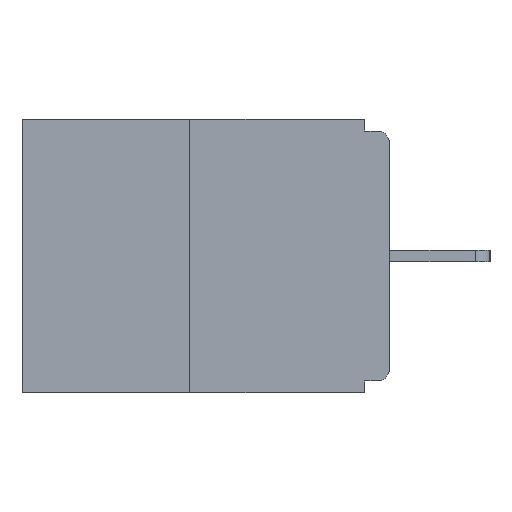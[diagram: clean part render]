
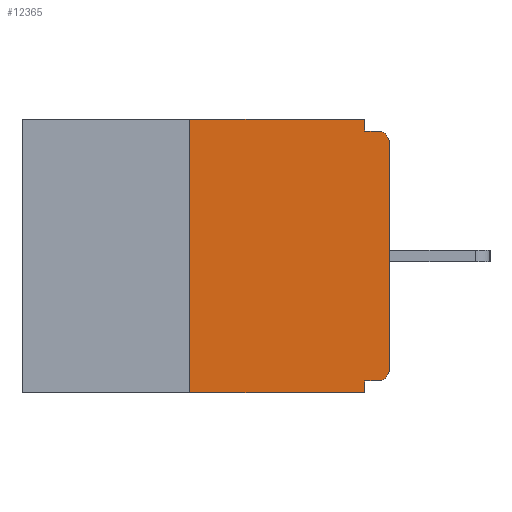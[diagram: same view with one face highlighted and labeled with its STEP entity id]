
A CAD part, left-side view. The second image highlights one B-rep face of the part: STEP entity #12365.
In plain terms, the highlighted planar face has unit normal (-1, 0, 0).
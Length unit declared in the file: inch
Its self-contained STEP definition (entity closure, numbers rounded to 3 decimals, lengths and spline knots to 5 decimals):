
#822 = DIRECTION ( 'NONE',  ( 0., 1., 0. ) ) ;
#905 = CARTESIAN_POINT ( 'NONE',  ( 0., 0.031, -0.015 ) ) ;
#998 = CARTESIAN_POINT ( 'NONE',  ( 0., 0.031, -0.343 ) ) ;
#1504 = DIRECTION ( 'NONE',  ( 0., -1., 0. ) ) ;
#1650 = VERTEX_POINT ( 'NONE', #905 ) ;
#1698 = CARTESIAN_POINT ( 'NONE',  ( 0., 0., -0.03 ) ) ;
#1766 = VERTEX_POINT ( 'NONE', #1698 ) ;
#1811 = EDGE_CURVE ( 'NONE', #2422, #1650, #21264, .T. ) ;
#2151 = EDGE_CURVE ( 'NONE', #22744, #8862, #3269, .T. ) ;
#2422 = VERTEX_POINT ( 'NONE', #18905 ) ;
#2938 = VECTOR ( 'NONE', #8432, 39.37008 ) ;
#3102 = EDGE_CURVE ( 'NONE', #8862, #6666, #23580, .T. ) ;
#3162 = CARTESIAN_POINT ( 'NONE',  ( 0., 0.015, -0.03 ) ) ;
#3269 = LINE ( 'NONE', #3898, #12607 ) ;
#3799 = LINE ( 'NONE', #23563, #12544 ) ;
#3820 = DIRECTION ( 'NONE',  ( 0., 0., -1. ) ) ;
#3898 = CARTESIAN_POINT ( 'NONE',  ( 0., 0., -0.328 ) ) ;
#4153 = DIRECTION ( 'NONE',  ( 0., 0., 1. ) ) ;
#4373 = EDGE_CURVE ( 'NONE', #10831, #6666, #16739, .T. ) ;
#4634 = EDGE_LOOP ( 'NONE', ( #5738, #5782, #6149, #6290, #6574, #6686, #6690, #6829, #7350, #7524 ) ) ;
#5040 = DIRECTION ( 'NONE',  ( 0., 0., -1. ) ) ;
#5623 = EDGE_CURVE ( 'NONE', #10831, #16930, #23477, .T. ) ;
#5738 = ORIENTED_EDGE ( 'NONE', *, *, #20176, .F. ) ;
#5782 = ORIENTED_EDGE ( 'NONE', *, *, #5623, .F. ) ;
#5790 = DIRECTION ( 'NONE',  ( 0., -1., 0. ) ) ;
#6149 = ORIENTED_EDGE ( 'NONE', *, *, #4373, .T. ) ;
#6290 = ORIENTED_EDGE ( 'NONE', *, *, #3102, .F. ) ;
#6547 = CARTESIAN_POINT ( 'NONE',  ( 0., 0., -0.015 ) ) ;
#6574 = ORIENTED_EDGE ( 'NONE', *, *, #2151, .F. ) ;
#6611 = VECTOR ( 'NONE', #22834, 39.37008 ) ;
#6666 = VERTEX_POINT ( 'NONE', #20913 ) ;
#6686 = ORIENTED_EDGE ( 'NONE', *, *, #17484, .T. ) ;
#6690 = ORIENTED_EDGE ( 'NONE', *, *, #7205, .T. ) ;
#6764 = DIRECTION ( 'NONE',  ( 0., 0., 1. ) ) ;
#6829 = ORIENTED_EDGE ( 'NONE', *, *, #15104, .T. ) ;
#7196 = CARTESIAN_POINT ( 'NONE',  ( 0., 0.46, 0. ) ) ;
#7205 = EDGE_CURVE ( 'NONE', #22937, #1766, #16019, .T. ) ;
#7350 = ORIENTED_EDGE ( 'NONE', *, *, #19973, .F. ) ;
#7524 = ORIENTED_EDGE ( 'NONE', *, *, #1811, .F. ) ;
#7939 = AXIS2_PLACEMENT_3D ( 'NONE', #3162, #16099, #5040 ) ;
#8432 = DIRECTION ( 'NONE',  ( 0., -1., 0. ) ) ;
#8862 = VERTEX_POINT ( 'NONE', #17153 ) ;
#8929 = FACE_OUTER_BOUND ( 'NONE', #4634, .T. ) ;
#8953 = DIRECTION ( 'NONE',  ( -1., 0., 0. ) ) ;
#9081 = DIRECTION ( 'NONE',  ( 0., 0., -1. ) ) ;
#10043 = CARTESIAN_POINT ( 'NONE',  ( 0., 0.25, -0.343 ) ) ;
#10435 = CARTESIAN_POINT ( 'NONE',  ( 0., 0.25, 0. ) ) ;
#10768 = VECTOR ( 'NONE', #5790, 39.37008 ) ;
#10831 = VERTEX_POINT ( 'NONE', #10043 ) ;
#12298 = CARTESIAN_POINT ( 'NONE',  ( 0., 0.25, 0. ) ) ;
#12365 = ADVANCED_FACE ( 'NONE', ( #8929 ), #12728, .F. ) ;
#12544 = VECTOR ( 'NONE', #1504, 39.37008 ) ;
#12607 = VECTOR ( 'NONE', #822, 39.37008 ) ;
#12728 = PLANE ( 'NONE',  #23051 ) ;
#12901 = CARTESIAN_POINT ( 'NONE',  ( 0., 0.031, 0. ) ) ;
#12955 = AXIS2_PLACEMENT_3D ( 'NONE', #19921, #8953, #21729 ) ;
#13418 = VECTOR ( 'NONE', #3820, 39.37008 ) ;
#13444 = CARTESIAN_POINT ( 'NONE',  ( 0., 0., 0. ) ) ;
#13465 = LINE ( 'NONE', #6547, #2938 ) ;
#13819 = CARTESIAN_POINT ( 'NONE',  ( 0., 0.015, -0.015 ) ) ;
#14599 = CARTESIAN_POINT ( 'NONE',  ( 0., 0.46, -0.343 ) ) ;
#15104 = EDGE_CURVE ( 'NONE', #1766, #21545, #17030, .T. ) ;
#15406 = CARTESIAN_POINT ( 'NONE',  ( 0., 0., -0.313 ) ) ;
#15467 = VECTOR ( 'NONE', #4153, 39.37008 ) ;
#16019 = LINE ( 'NONE', #13444, #15467 ) ;
#16099 = DIRECTION ( 'NONE',  ( -1., 0., 0. ) ) ;
#16739 = LINE ( 'NONE', #14599, #10768 ) ;
#16930 = VERTEX_POINT ( 'NONE', #10435 ) ;
#17030 = CIRCLE ( 'NONE', #7939, 0.015 ) ;
#17153 = CARTESIAN_POINT ( 'NONE',  ( 0., 0.031, -0.328 ) ) ;
#17484 = EDGE_CURVE ( 'NONE', #22744, #22937, #20077, .T. ) ;
#18905 = CARTESIAN_POINT ( 'NONE',  ( 0., 0.031, 0. ) ) ;
#19921 = CARTESIAN_POINT ( 'NONE',  ( 0., 0.015, -0.313 ) ) ;
#19973 = EDGE_CURVE ( 'NONE', #1650, #21545, #13465, .T. ) ;
#20041 = DIRECTION ( 'NONE',  ( 1., 0., 0. ) ) ;
#20077 = CIRCLE ( 'NONE', #12955, 0.015 ) ;
#20176 = EDGE_CURVE ( 'NONE', #16930, #2422, #3799, .T. ) ;
#20425 = CARTESIAN_POINT ( 'NONE',  ( 0., 0.015, -0.328 ) ) ;
#20913 = CARTESIAN_POINT ( 'NONE',  ( 0., 0.031, -0.343 ) ) ;
#21264 = LINE ( 'NONE', #12901, #6611 ) ;
#21545 = VERTEX_POINT ( 'NONE', #13819 ) ;
#21729 = DIRECTION ( 'NONE',  ( 0., 0., -1. ) ) ;
#22744 = VERTEX_POINT ( 'NONE', #20425 ) ;
#22834 = DIRECTION ( 'NONE',  ( 0., 0., -1. ) ) ;
#22925 = VECTOR ( 'NONE', #6764, 39.37008 ) ;
#22937 = VERTEX_POINT ( 'NONE', #15406 ) ;
#23051 = AXIS2_PLACEMENT_3D ( 'NONE', #7196, #20041, #9081 ) ;
#23477 = LINE ( 'NONE', #12298, #22925 ) ;
#23563 = CARTESIAN_POINT ( 'NONE',  ( 0., 0.46, 0. ) ) ;
#23580 = LINE ( 'NONE', #998, #13418 ) ;
